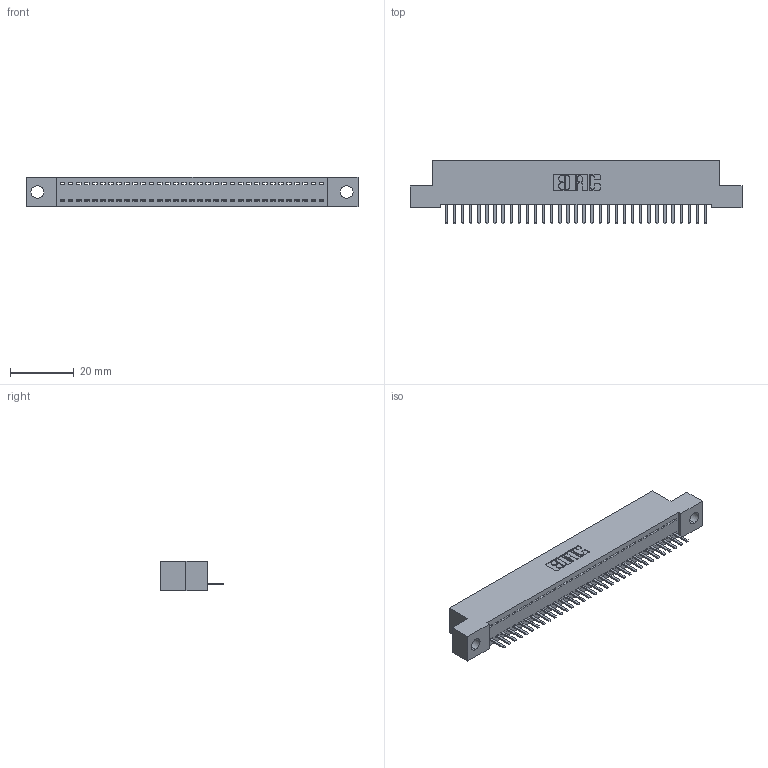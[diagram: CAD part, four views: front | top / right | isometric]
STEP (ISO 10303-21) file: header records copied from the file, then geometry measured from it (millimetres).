
FILE_DESCRIPTION (( 'STEP AP203' ), '1' );
FILE_NAME ('392-033-520-104.STEP', '2019-10-07T15:08:11', ( '' ), ( '' ), 'SwSTEP 2.0', 'SolidWorks 2016', '' );
FILE_SCHEMA (( 'CONFIG_CONTROL_DESIGN' ));
Length unit declared in the file: inch
Products named in the file (3): 342 Part_.156 TH; 345-292-001_345-293-120; 392-033-520-104
Assembly tree (34 placements, depth 2):
  392-033-520-104
    342 Part_.156 TH
    345-292-001_345-293-120  x33
Bounding box: 104.14 x 20.02 x 9.4 mm (x, y, z)
Volume: 8915.9 mm3; surface area: 12439.7 mm2
Topology: 34 solids, 34 shells, 2156 faces, 6371 edges, 4158 vertices
Faces by surface type: plane 1518, cylinder 638
Entity records: 21323 total; most frequent: CARTESIAN_POINT 3697, ORIENTED_EDGE 3654, DIRECTION 3125, EDGE_CURVE 1827, LINE 1695, VECTOR 1695, VERTEX_POINT 1214, AXIS2_PLACEMENT_3D 715
